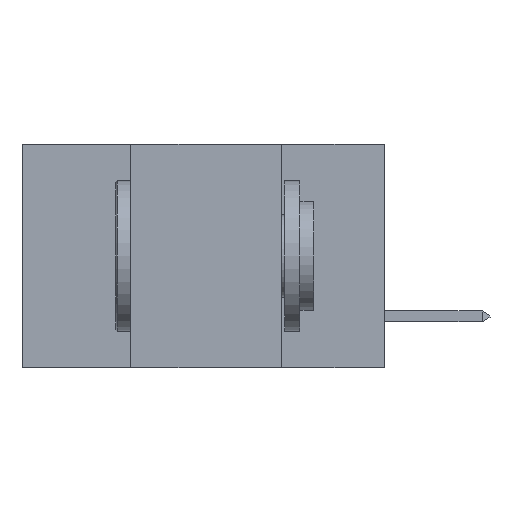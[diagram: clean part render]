
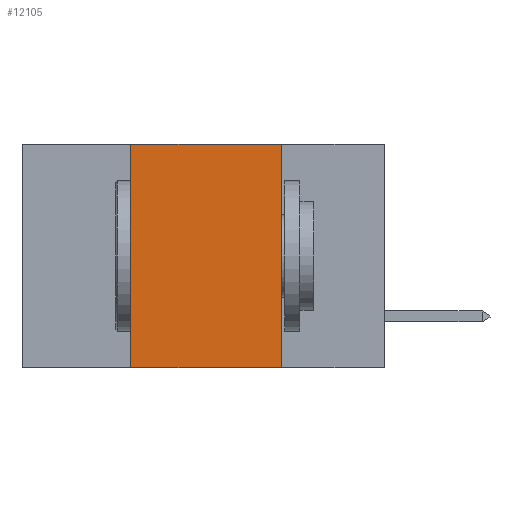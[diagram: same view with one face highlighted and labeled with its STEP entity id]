
A CAD part, left-side view. The second image highlights one B-rep face of the part: STEP entity #12105.
In plain terms, the highlighted planar face has unit normal (-1, 0, 0).
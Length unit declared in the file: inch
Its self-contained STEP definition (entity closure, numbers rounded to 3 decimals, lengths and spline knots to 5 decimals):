
#502 = VERTEX_POINT ( 'NONE', #14501 ) ;
#1424 = VERTEX_POINT ( 'NONE', #11167 ) ;
#2657 = EDGE_CURVE ( 'NONE', #11486, #1424, #5407, .T. ) ;
#2718 = DIRECTION ( 'NONE',  ( 0., -1., 0. ) ) ;
#2846 = VECTOR ( 'NONE', #3627, 39.37008 ) ;
#2869 = CARTESIAN_POINT ( 'NONE',  ( 0., 0.6, -0.37 ) ) ;
#2879 = CARTESIAN_POINT ( 'NONE',  ( 0., 0.6, 0. ) ) ;
#2895 = CARTESIAN_POINT ( 'NONE',  ( 0., 0.42, 0. ) ) ;
#3388 = LINE ( 'NONE', #7851, #12027 ) ;
#3627 = DIRECTION ( 'NONE',  ( 0., 0., -1. ) ) ;
#3785 = VERTEX_POINT ( 'NONE', #9764 ) ;
#3979 = DIRECTION ( 'NONE',  ( 1., 0., 0. ) ) ;
#4476 = FACE_OUTER_BOUND ( 'NONE', #5786, .T. ) ;
#4589 = CARTESIAN_POINT ( 'NONE',  ( 0., 0.6, 0. ) ) ;
#4715 = EDGE_CURVE ( 'NONE', #3785, #502, #13851, .T. ) ;
#5407 = LINE ( 'NONE', #4589, #11103 ) ;
#5461 = LINE ( 'NONE', #7131, #2846 ) ;
#5483 = EDGE_CURVE ( 'NONE', #3785, #11486, #3388, .T. ) ;
#5786 = EDGE_LOOP ( 'NONE', ( #11310, #14124, #11658, #6719 ) ) ;
#6210 = AXIS2_PLACEMENT_3D ( 'NONE', #2879, #3979, #11893 ) ;
#6250 = EDGE_CURVE ( 'NONE', #1424, #502, #5461, .T. ) ;
#6719 = ORIENTED_EDGE ( 'NONE', *, *, #4715, .T. ) ;
#7131 = CARTESIAN_POINT ( 'NONE',  ( 0., 0.17, 0. ) ) ;
#7851 = CARTESIAN_POINT ( 'NONE',  ( 0., 0.42, 0. ) ) ;
#7942 = DIRECTION ( 'NONE',  ( 0., 0., 1. ) ) ;
#9632 = PLANE ( 'NONE',  #6210 ) ;
#9764 = CARTESIAN_POINT ( 'NONE',  ( 0., 0.42, -0.37 ) ) ;
#10691 = VECTOR ( 'NONE', #2718, 39.37008 ) ;
#11103 = VECTOR ( 'NONE', #14351, 39.37008 ) ;
#11167 = CARTESIAN_POINT ( 'NONE',  ( 0., 0.17, 0. ) ) ;
#11310 = ORIENTED_EDGE ( 'NONE', *, *, #6250, .F. ) ;
#11486 = VERTEX_POINT ( 'NONE', #2895 ) ;
#11658 = ORIENTED_EDGE ( 'NONE', *, *, #5483, .F. ) ;
#11893 = DIRECTION ( 'NONE',  ( 0., 0., -1. ) ) ;
#12027 = VECTOR ( 'NONE', #7942, 39.37008 ) ;
#12105 = ADVANCED_FACE ( 'NONE', ( #4476 ), #9632, .F. ) ;
#13851 = LINE ( 'NONE', #2869, #10691 ) ;
#14124 = ORIENTED_EDGE ( 'NONE', *, *, #2657, .F. ) ;
#14351 = DIRECTION ( 'NONE',  ( 0., -1., 0. ) ) ;
#14501 = CARTESIAN_POINT ( 'NONE',  ( 0., 0.17, -0.37 ) ) ;
